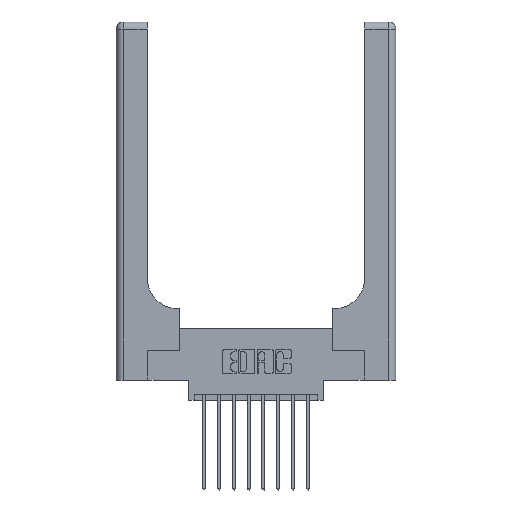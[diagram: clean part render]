
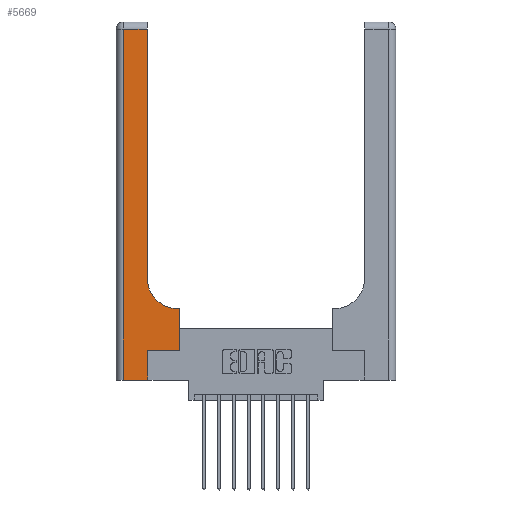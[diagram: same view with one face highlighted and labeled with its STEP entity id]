
A CAD part, top view. The second image highlights one B-rep face of the part: STEP entity #5669.
In plain terms, the highlighted planar face has unit normal (0, 0, 1).
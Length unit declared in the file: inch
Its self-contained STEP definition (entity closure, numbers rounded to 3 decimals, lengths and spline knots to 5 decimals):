
#144 = CIRCLE ( 'NONE', #4412, 0.25 ) ;
#307 = VERTEX_POINT ( 'NONE', #8314 ) ;
#548 = DIRECTION ( 'NONE',  ( 0., 0., -1. ) ) ;
#757 = VERTEX_POINT ( 'NONE', #1062 ) ;
#1051 = CARTESIAN_POINT ( 'NONE',  ( 0.06, 3., 0.37 ) ) ;
#1062 = CARTESIAN_POINT ( 'NONE',  ( 0.51, 0.6, 0.37 ) ) ;
#1127 = DIRECTION ( 'NONE',  ( 0., -1., 0. ) ) ;
#1167 = VECTOR ( 'NONE', #13439, 39.37008 ) ;
#1244 = VERTEX_POINT ( 'NONE', #14030 ) ;
#1255 = VERTEX_POINT ( 'NONE', #5359 ) ;
#1272 = CARTESIAN_POINT ( 'NONE',  ( 0., 0., 0.37 ) ) ;
#1544 = CARTESIAN_POINT ( 'NONE',  ( 0., 3., 0.37 ) ) ;
#1910 = DIRECTION ( 'NONE',  ( 0., 1., 0. ) ) ;
#2107 = LINE ( 'NONE', #7107, #6267 ) ;
#2213 = CARTESIAN_POINT ( 'NONE',  ( 0., 2.94, 0.37 ) ) ;
#2372 = ORIENTED_EDGE ( 'NONE', *, *, #8495, .T. ) ;
#2456 = LINE ( 'NONE', #1272, #5513 ) ;
#2606 = VECTOR ( 'NONE', #1127, 39.37008 ) ;
#2614 = ORIENTED_EDGE ( 'NONE', *, *, #4257, .T. ) ;
#2655 = VECTOR ( 'NONE', #1910, 39.37008 ) ;
#3014 = EDGE_CURVE ( 'NONE', #9283, #1255, #13367, .T. ) ;
#3423 = ORIENTED_EDGE ( 'NONE', *, *, #13972, .T. ) ;
#3999 = VERTEX_POINT ( 'NONE', #15434 ) ;
#4006 = ORIENTED_EDGE ( 'NONE', *, *, #11342, .T. ) ;
#4021 = ORIENTED_EDGE ( 'NONE', *, *, #8928, .T. ) ;
#4209 = DIRECTION ( 'NONE',  ( 0., 0., -1. ) ) ;
#4257 = EDGE_CURVE ( 'NONE', #1244, #307, #13371, .T. ) ;
#4412 = AXIS2_PLACEMENT_3D ( 'NONE', #7618, #548, #9200 ) ;
#4450 = LINE ( 'NONE', #11620, #15552 ) ;
#5359 = CARTESIAN_POINT ( 'NONE',  ( 0.528, 0.25, 0.37 ) ) ;
#5513 = VECTOR ( 'NONE', #6060, 39.37008 ) ;
#5669 = ADVANCED_FACE ( 'NONE', ( #10098 ), #12401, .F. ) ;
#6060 = DIRECTION ( 'NONE',  ( 1., 0., 0. ) ) ;
#6108 = CARTESIAN_POINT ( 'NONE',  ( 0.528, 0.6, 0.37 ) ) ;
#6125 = CARTESIAN_POINT ( 'NONE',  ( 0.26, 3., 0.37 ) ) ;
#6267 = VECTOR ( 'NONE', #12957, 39.37008 ) ;
#6610 = LINE ( 'NONE', #11414, #2655 ) ;
#7107 = CARTESIAN_POINT ( 'NONE',  ( 0.528, 0.25, 0.37 ) ) ;
#7127 = VECTOR ( 'NONE', #14321, 39.37008 ) ;
#7138 = EDGE_CURVE ( 'NONE', #15494, #757, #4450, .T. ) ;
#7618 = CARTESIAN_POINT ( 'NONE',  ( 0.51, 0.85, 0.37 ) ) ;
#8286 = EDGE_CURVE ( 'NONE', #13725, #3999, #2456, .T. ) ;
#8314 = CARTESIAN_POINT ( 'NONE',  ( 0.26, 2.94, 0.37 ) ) ;
#8495 = EDGE_CURVE ( 'NONE', #1255, #15494, #2107, .T. ) ;
#8682 = VECTOR ( 'NONE', #13522, 39.37008 ) ;
#8722 = CARTESIAN_POINT ( 'NONE',  ( 0.06, 0., 0.37 ) ) ;
#8917 = EDGE_CURVE ( 'NONE', #757, #1244, #144, .T. ) ;
#8928 = EDGE_CURVE ( 'NONE', #3999, #9283, #6610, .T. ) ;
#9200 = DIRECTION ( 'NONE',  ( 1., 0., 0. ) ) ;
#9251 = DIRECTION ( 'NONE',  ( -1., 0., 0. ) ) ;
#9283 = VERTEX_POINT ( 'NONE', #13734 ) ;
#10003 = CARTESIAN_POINT ( 'NONE',  ( 0.06, 2.94, 0.37 ) ) ;
#10098 = FACE_OUTER_BOUND ( 'NONE', #12436, .T. ) ;
#10185 = DIRECTION ( 'NONE',  ( -1., 0., 0. ) ) ;
#10403 = LINE ( 'NONE', #1051, #2606 ) ;
#10450 = LINE ( 'NONE', #2213, #7127 ) ;
#11290 = ORIENTED_EDGE ( 'NONE', *, *, #3014, .T. ) ;
#11342 = EDGE_CURVE ( 'NONE', #12327, #13725, #10403, .T. ) ;
#11414 = CARTESIAN_POINT ( 'NONE',  ( 0.265, 0., 0.37 ) ) ;
#11620 = CARTESIAN_POINT ( 'NONE',  ( 0.26, 0.6, 0.37 ) ) ;
#11669 = ORIENTED_EDGE ( 'NONE', *, *, #7138, .T. ) ;
#12105 = CARTESIAN_POINT ( 'NONE',  ( 0.265, 0.25, 0.37 ) ) ;
#12327 = VERTEX_POINT ( 'NONE', #10003 ) ;
#12374 = ORIENTED_EDGE ( 'NONE', *, *, #8917, .T. ) ;
#12401 = PLANE ( 'NONE',  #13740 ) ;
#12436 = EDGE_LOOP ( 'NONE', ( #2614, #3423, #4006, #14212, #4021, #11290, #2372, #11669, #12374 ) ) ;
#12957 = DIRECTION ( 'NONE',  ( 0., 1., 0. ) ) ;
#13367 = LINE ( 'NONE', #12105, #1167 ) ;
#13371 = LINE ( 'NONE', #6125, #8682 ) ;
#13439 = DIRECTION ( 'NONE',  ( 1., 0., 0. ) ) ;
#13522 = DIRECTION ( 'NONE',  ( 0., 1., 0. ) ) ;
#13725 = VERTEX_POINT ( 'NONE', #8722 ) ;
#13734 = CARTESIAN_POINT ( 'NONE',  ( 0.265, 0.25, 0.37 ) ) ;
#13740 = AXIS2_PLACEMENT_3D ( 'NONE', #1544, #4209, #10185 ) ;
#13972 = EDGE_CURVE ( 'NONE', #307, #12327, #10450, .T. ) ;
#14030 = CARTESIAN_POINT ( 'NONE',  ( 0.26, 0.85, 0.37 ) ) ;
#14212 = ORIENTED_EDGE ( 'NONE', *, *, #8286, .T. ) ;
#14321 = DIRECTION ( 'NONE',  ( -1., 0., 0. ) ) ;
#15434 = CARTESIAN_POINT ( 'NONE',  ( 0.265, 0., 0.37 ) ) ;
#15494 = VERTEX_POINT ( 'NONE', #6108 ) ;
#15552 = VECTOR ( 'NONE', #9251, 39.37008 ) ;
